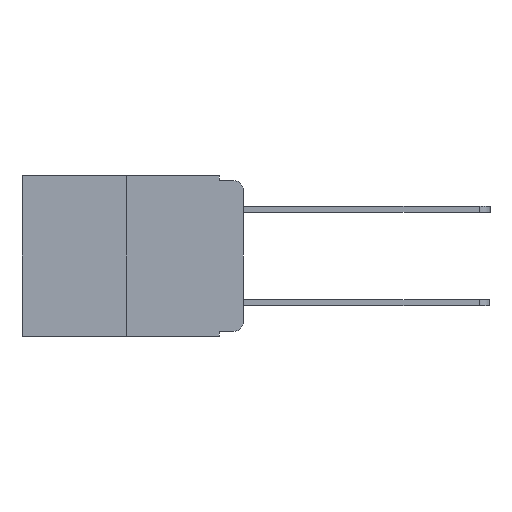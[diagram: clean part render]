
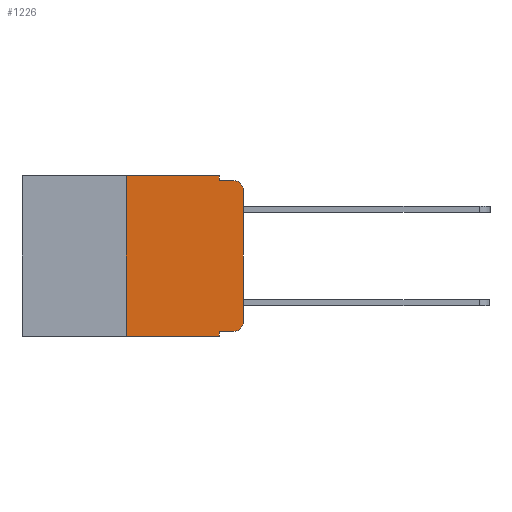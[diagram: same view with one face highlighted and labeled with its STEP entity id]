
A CAD part, left-side view. The second image highlights one B-rep face of the part: STEP entity #1226.
In plain terms, the highlighted planar face has unit normal (-1, 0, 0).
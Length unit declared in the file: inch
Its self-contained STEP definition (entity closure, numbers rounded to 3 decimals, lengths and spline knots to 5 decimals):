
#341 = DIRECTION ( 'NONE',  ( -1., 0., 0. ) ) ;
#350 = EDGE_CURVE ( 'NONE', #7001, #15595, #17608, .T. ) ;
#570 = DIRECTION ( 'NONE',  ( 0., -1., 0. ) ) ;
#706 = LINE ( 'NONE', #13025, #13357 ) ;
#715 = VERTEX_POINT ( 'NONE', #12276 ) ;
#926 = CARTESIAN_POINT ( 'NONE',  ( 0., 0., -0.03 ) ) ;
#1134 = CARTESIAN_POINT ( 'NONE',  ( 0., 0.051, 0. ) ) ;
#1226 = ADVANCED_FACE ( 'NONE', ( #7362 ), #9461, .F. ) ;
#1401 = VECTOR ( 'NONE', #15309, 39.37008 ) ;
#1408 = VERTEX_POINT ( 'NONE', #1134 ) ;
#1532 = ORIENTED_EDGE ( 'NONE', *, *, #6983, .T. ) ;
#1569 = DIRECTION ( 'NONE',  ( 0., -1., 0. ) ) ;
#2378 = EDGE_CURVE ( 'NONE', #5096, #7019, #19565, .T. ) ;
#2394 = DIRECTION ( 'NONE',  ( 0., 0., -1. ) ) ;
#2436 = LINE ( 'NONE', #10180, #18756 ) ;
#2768 = DIRECTION ( 'NONE',  ( 0., 0., -1. ) ) ;
#2795 = EDGE_CURVE ( 'NONE', #3508, #15595, #16824, .T. ) ;
#2938 = LINE ( 'NONE', #13829, #1401 ) ;
#3304 = CARTESIAN_POINT ( 'NONE',  ( 0., 0., -0.313 ) ) ;
#3508 = VERTEX_POINT ( 'NONE', #6587 ) ;
#3879 = VECTOR ( 'NONE', #8254, 39.37008 ) ;
#3954 = ORIENTED_EDGE ( 'NONE', *, *, #350, .T. ) ;
#4316 = DIRECTION ( 'NONE',  ( 0., 0., -1. ) ) ;
#4406 = LINE ( 'NONE', #6645, #3879 ) ;
#4559 = VECTOR ( 'NONE', #2768, 39.37008 ) ;
#5096 = VERTEX_POINT ( 'NONE', #926 ) ;
#5232 = EDGE_LOOP ( 'NONE', ( #1532, #17355, #6530, #13844, #19563, #15160, #3954, #8493, #5724, #18134 ) ) ;
#5390 = EDGE_CURVE ( 'NONE', #715, #1408, #2436, .T. ) ;
#5724 = ORIENTED_EDGE ( 'NONE', *, *, #13982, .T. ) ;
#6128 = CARTESIAN_POINT ( 'NONE',  ( 0., 0.051, -0.343 ) ) ;
#6530 = ORIENTED_EDGE ( 'NONE', *, *, #19393, .F. ) ;
#6587 = CARTESIAN_POINT ( 'NONE',  ( 0., 0.051, -0.333 ) ) ;
#6645 = CARTESIAN_POINT ( 'NONE',  ( 0., 0.051, -0.01 ) ) ;
#6983 = EDGE_CURVE ( 'NONE', #19345, #5096, #10331, .T. ) ;
#7001 = VERTEX_POINT ( 'NONE', #8129 ) ;
#7019 = VERTEX_POINT ( 'NONE', #8205 ) ;
#7362 = FACE_OUTER_BOUND ( 'NONE', #5232, .T. ) ;
#8129 = CARTESIAN_POINT ( 'NONE',  ( 0., 0.25, -0.343 ) ) ;
#8205 = CARTESIAN_POINT ( 'NONE',  ( 0., 0.02, -0.01 ) ) ;
#8254 = DIRECTION ( 'NONE',  ( 0., -1., 0. ) ) ;
#8493 = ORIENTED_EDGE ( 'NONE', *, *, #2795, .F. ) ;
#8624 = CIRCLE ( 'NONE', #16057, 0.02 ) ;
#8949 = AXIS2_PLACEMENT_3D ( 'NONE', #11697, #12515, #4316 ) ;
#8979 = CARTESIAN_POINT ( 'NONE',  ( 0., 0.051, -0.01 ) ) ;
#9110 = AXIS2_PLACEMENT_3D ( 'NONE', #19765, #16842, #2394 ) ;
#9461 = PLANE ( 'NONE',  #8949 ) ;
#9979 = CARTESIAN_POINT ( 'NONE',  ( 0., 0.02, -0.313 ) ) ;
#10061 = EDGE_CURVE ( 'NONE', #1408, #11141, #10830, .T. ) ;
#10180 = CARTESIAN_POINT ( 'NONE',  ( 0., 0.473, 0. ) ) ;
#10331 = LINE ( 'NONE', #20062, #14394 ) ;
#10830 = LINE ( 'NONE', #10909, #18299 ) ;
#10909 = CARTESIAN_POINT ( 'NONE',  ( 0., 0.051, 0. ) ) ;
#11141 = VERTEX_POINT ( 'NONE', #8979 ) ;
#11504 = DIRECTION ( 'NONE',  ( 0., 0., -1. ) ) ;
#11536 = EDGE_CURVE ( 'NONE', #12313, #19345, #8624, .T. ) ;
#11697 = CARTESIAN_POINT ( 'NONE',  ( 0., 0.473, 0. ) ) ;
#12276 = CARTESIAN_POINT ( 'NONE',  ( 0., 0.25, 0. ) ) ;
#12313 = VERTEX_POINT ( 'NONE', #18057 ) ;
#12515 = DIRECTION ( 'NONE',  ( 1., 0., 0. ) ) ;
#12752 = DIRECTION ( 'NONE',  ( 0., 0., 1. ) ) ;
#13025 = CARTESIAN_POINT ( 'NONE',  ( 0., 0.051, -0.333 ) ) ;
#13357 = VECTOR ( 'NONE', #14528, 39.37008 ) ;
#13829 = CARTESIAN_POINT ( 'NONE',  ( 0., 0.25, 0. ) ) ;
#13844 = ORIENTED_EDGE ( 'NONE', *, *, #10061, .F. ) ;
#13982 = EDGE_CURVE ( 'NONE', #3508, #12313, #706, .T. ) ;
#14394 = VECTOR ( 'NONE', #12752, 39.37008 ) ;
#14528 = DIRECTION ( 'NONE',  ( 0., -1., 0. ) ) ;
#15160 = ORIENTED_EDGE ( 'NONE', *, *, #18072, .F. ) ;
#15309 = DIRECTION ( 'NONE',  ( 0., 0., 1. ) ) ;
#15595 = VERTEX_POINT ( 'NONE', #6128 ) ;
#15717 = CARTESIAN_POINT ( 'NONE',  ( 0., 0.473, -0.343 ) ) ;
#16057 = AXIS2_PLACEMENT_3D ( 'NONE', #9979, #341, #11504 ) ;
#16824 = LINE ( 'NONE', #19444, #4559 ) ;
#16842 = DIRECTION ( 'NONE',  ( -1., 0., 0. ) ) ;
#16864 = DIRECTION ( 'NONE',  ( 0., 0., -1. ) ) ;
#17355 = ORIENTED_EDGE ( 'NONE', *, *, #2378, .T. ) ;
#17608 = LINE ( 'NONE', #15717, #18077 ) ;
#18057 = CARTESIAN_POINT ( 'NONE',  ( 0., 0.02, -0.333 ) ) ;
#18072 = EDGE_CURVE ( 'NONE', #7001, #715, #2938, .T. ) ;
#18077 = VECTOR ( 'NONE', #1569, 39.37008 ) ;
#18134 = ORIENTED_EDGE ( 'NONE', *, *, #11536, .T. ) ;
#18299 = VECTOR ( 'NONE', #16864, 39.37008 ) ;
#18756 = VECTOR ( 'NONE', #570, 39.37008 ) ;
#19345 = VERTEX_POINT ( 'NONE', #3304 ) ;
#19393 = EDGE_CURVE ( 'NONE', #11141, #7019, #4406, .T. ) ;
#19444 = CARTESIAN_POINT ( 'NONE',  ( 0., 0.051, 0. ) ) ;
#19563 = ORIENTED_EDGE ( 'NONE', *, *, #5390, .F. ) ;
#19565 = CIRCLE ( 'NONE', #9110, 0.02 ) ;
#19765 = CARTESIAN_POINT ( 'NONE',  ( 0., 0.02, -0.03 ) ) ;
#20062 = CARTESIAN_POINT ( 'NONE',  ( 0., 0., 0. ) ) ;
